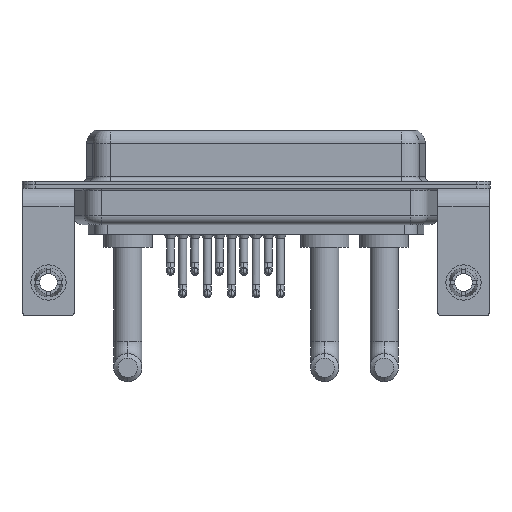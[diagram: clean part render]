
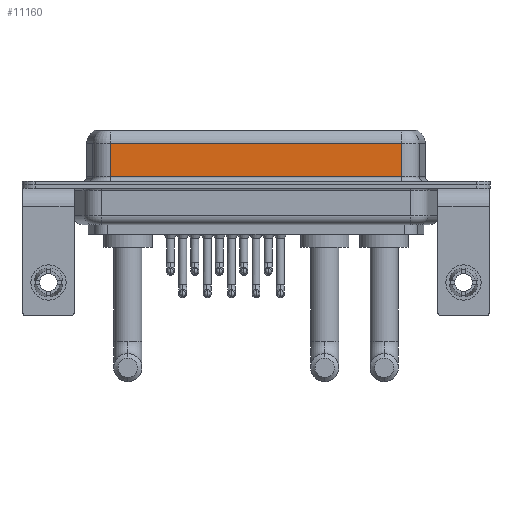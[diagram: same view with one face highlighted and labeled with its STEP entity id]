
A CAD part, front view. The second image highlights one B-rep face of the part: STEP entity #11160.
In plain terms, the highlighted planar face has unit normal (0, -1, 0).
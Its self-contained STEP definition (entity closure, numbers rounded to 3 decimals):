
#467 = CARTESIAN_POINT ( 'NONE',  ( 40.037, -3.95, 0.9 ) ) ;
#1801 = EDGE_CURVE ( 'NONE', #15617, #10814, #13622, .T. ) ;
#2987 = EDGE_CURVE ( 'NONE', #4354, #15617, #19702, .T. ) ;
#3182 = CARTESIAN_POINT ( 'NONE',  ( 7.013, -3.95, 6.4 ) ) ;
#3913 = VECTOR ( 'NONE', #19677, 1000. ) ;
#3976 = AXIS2_PLACEMENT_3D ( 'NONE', #15477, #13747, #18732 ) ;
#4076 = CARTESIAN_POINT ( 'NONE',  ( 7.013, -3.95, 0.9 ) ) ;
#4354 = VERTEX_POINT ( 'NONE', #13002 ) ;
#5191 = ORIENTED_EDGE ( 'NONE', *, *, #1801, .T. ) ;
#6306 = EDGE_CURVE ( 'NONE', #16563, #4354, #16229, .T. ) ;
#7102 = DIRECTION ( 'NONE',  ( 1., 0., 0. ) ) ;
#7668 = VECTOR ( 'NONE', #7970, 1000. ) ;
#7970 = DIRECTION ( 'NONE',  ( -1., 0., 0. ) ) ;
#8027 = ORIENTED_EDGE ( 'NONE', *, *, #2987, .T. ) ;
#8300 = EDGE_CURVE ( 'NONE', #16563, #10814, #14372, .T. ) ;
#9097 = VECTOR ( 'NONE', #7102, 1000. ) ;
#10044 = DIRECTION ( 'NONE',  ( 0., 0., -1. ) ) ;
#10814 = VERTEX_POINT ( 'NONE', #12147 ) ;
#10920 = ORIENTED_EDGE ( 'NONE', *, *, #8300, .F. ) ;
#11121 = CARTESIAN_POINT ( 'NONE',  ( 40.037, -3.95, 6.4 ) ) ;
#11160 = ADVANCED_FACE ( 'NONE', ( #19054 ), #15686, .F. ) ;
#11678 = CARTESIAN_POINT ( 'NONE',  ( 40.037, -3.95, 4.65 ) ) ;
#12147 = CARTESIAN_POINT ( 'NONE',  ( 40.037, -3.95, 0.9 ) ) ;
#13002 = CARTESIAN_POINT ( 'NONE',  ( 7.013, -3.95, 4.65 ) ) ;
#13622 = LINE ( 'NONE', #467, #9097 ) ;
#13747 = DIRECTION ( 'NONE',  ( 0., 1., 0. ) ) ;
#14372 = LINE ( 'NONE', #11121, #3913 ) ;
#15477 = CARTESIAN_POINT ( 'NONE',  ( 40.037, -3.95, 6.4 ) ) ;
#15617 = VERTEX_POINT ( 'NONE', #4076 ) ;
#15686 = PLANE ( 'NONE',  #3976 ) ;
#16006 = VECTOR ( 'NONE', #10044, 1000. ) ;
#16085 = ORIENTED_EDGE ( 'NONE', *, *, #6306, .T. ) ;
#16229 = LINE ( 'NONE', #11678, #7668 ) ;
#16563 = VERTEX_POINT ( 'NONE', #19540 ) ;
#18732 = DIRECTION ( 'NONE',  ( 0., 0., 1. ) ) ;
#19054 = FACE_OUTER_BOUND ( 'NONE', #21140, .T. ) ;
#19540 = CARTESIAN_POINT ( 'NONE',  ( 40.037, -3.95, 4.65 ) ) ;
#19677 = DIRECTION ( 'NONE',  ( 0., 0., -1. ) ) ;
#19702 = LINE ( 'NONE', #3182, #16006 ) ;
#21140 = EDGE_LOOP ( 'NONE', ( #10920, #16085, #8027, #5191 ) ) ;
